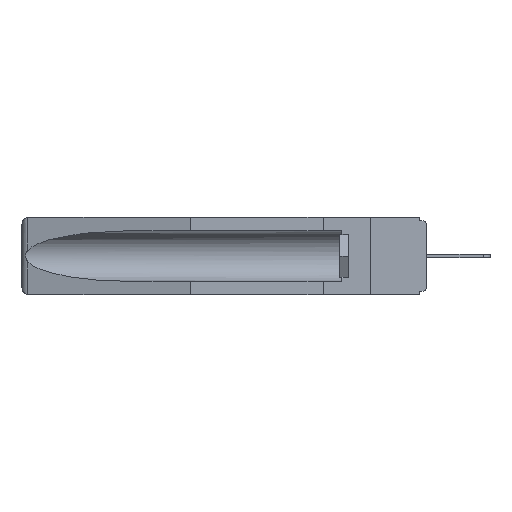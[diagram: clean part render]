
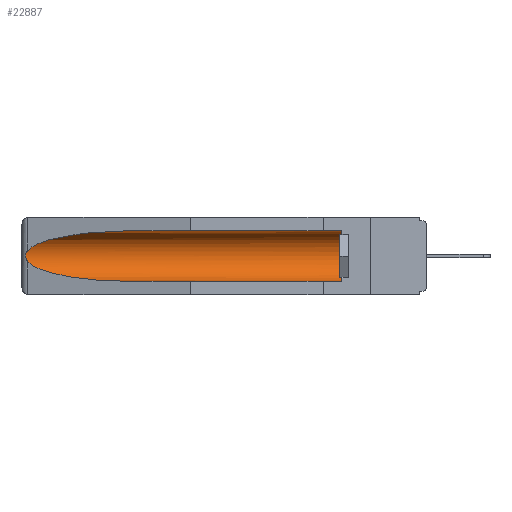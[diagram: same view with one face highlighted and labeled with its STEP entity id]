
A CAD part, left-side view. The second image highlights one B-rep face of the part: STEP entity #22887.
In plain terms, the highlighted cylindrical face has radius 2.857 mm (diameter 5.715 mm), a partial arc.
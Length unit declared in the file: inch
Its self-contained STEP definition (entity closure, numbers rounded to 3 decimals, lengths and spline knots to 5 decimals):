
#917 = CARTESIAN_POINT ( 'NONE',  ( 0.155, -0.30754, -0.1715 ) ) ;
#987 = CARTESIAN_POINT ( 'NONE',  ( 0.2675, 1.53308, -0.16763 ) ) ;
#1352 = CARTESIAN_POINT ( 'NONE',  ( 0.21114, 1.30732, -0.284 ) ) ;
#1881 = ORIENTED_EDGE ( 'NONE', *, *, #13844, .T. ) ;
#3931 = ORIENTED_EDGE ( 'NONE', *, *, #7200, .T. ) ;
#4215 = CARTESIAN_POINT ( 'NONE',  ( 0.26537, 1.52718, -0.19328 ) ) ;
#4476 = DIRECTION ( 'NONE',  ( 0., 1., 0. ) ) ;
#4781 = CARTESIAN_POINT ( 'NONE',  ( 0.155, 0.126, -0.059 ) ) ;
#4835 = EDGE_CURVE ( 'NONE', #23965, #17262, #27785, .T. ) ;
#5038 = VERTEX_POINT ( 'NONE', #23030 ) ;
#5312 = ORIENTED_EDGE ( 'NONE', *, *, #16199, .T. ) ;
#5454 = LINE ( 'NONE', #9443, #24517 ) ;
#5993 = VECTOR ( 'NONE', #4476, 39.37008 ) ;
#6792 = EDGE_LOOP ( 'NONE', ( #22657, #1881, #5312, #8667, #3931, #7073 ) ) ;
#7031 = LINE ( 'NONE', #11035, #5993 ) ;
#7073 = ORIENTED_EDGE ( 'NONE', *, *, #25296, .T. ) ;
#7200 = EDGE_CURVE ( 'NONE', #24203, #20378, #25875, .T. ) ;
#7541 = CARTESIAN_POINT ( 'NONE',  ( 0.26537, 1.52718, -0.19328 ) ) ;
#7619 = DIRECTION ( 'NONE',  ( 0., 0., 1. ) ) ;
#7779 = CARTESIAN_POINT ( 'NONE',  ( 0.25451, 1.48313, -0.24835 ) ) ;
#8667 = ORIENTED_EDGE ( 'NONE', *, *, #20708, .F. ) ;
#9443 = CARTESIAN_POINT ( 'NONE',  ( 0.155, -0.30754, -0.059 ) ) ;
#9468 = CYLINDRICAL_SURFACE ( 'NONE', #20634, 0.1125 ) ;
#9616 = DIRECTION ( 'NONE',  ( 0., 1., 0. ) ) ;
#9686 = CARTESIAN_POINT ( 'NONE',  ( 0.2673, 1.53269, -0.17917 ) ) ;
#10258 = VERTEX_POINT ( 'NONE', #4215 ) ;
#11035 = CARTESIAN_POINT ( 'NONE',  ( 0.155, -0.30754, -0.284 ) ) ;
#11532 = CARTESIAN_POINT ( 'NONE',  ( 0.26597, 1.52961, -0.15275 ) ) ;
#12071 = CARTESIAN_POINT ( 'NONE',  ( 0.21114, 1.30732, -0.059 ) ) ;
#12356 = DIRECTION ( 'NONE',  ( 0., -1., 0. ) ) ;
#13382 = CARTESIAN_POINT ( 'NONE',  ( 0.26654, 1.53092, -0.15636 ) ) ;
#13660 = CARTESIAN_POINT ( 'NONE',  ( 0.155, 0.126, -0.284 ) ) ;
#13801 = CARTESIAN_POINT ( 'NONE',  ( 0.26537, 1.52718, -0.14972 ) ) ;
#13844 = EDGE_CURVE ( 'NONE', #17262, #10258, #16326, .T. ) ;
#13860 = DIRECTION ( 'NONE',  ( 0., 1., 0. ) ) ;
#16199 = EDGE_CURVE ( 'NONE', #10258, #5038, #18138, .T. ) ;
#16209 = CARTESIAN_POINT ( 'NONE',  ( 0.25451, 1.48313, -0.09465 ) ) ;
#16326 = B_SPLINE_CURVE_WITH_KNOTS ( 'NONE', 3,
 ( #18217, #11532, #13382, #27038, #987, #20061, #9686, #17784, #18070, #7541 ),
 .UNSPECIFIED., .F., .F.,
 ( 4, 2, 2, 2, 4 ),
 ( 0., 0.00029, 0.00058, 0.00087, 0.00117 ),
 .UNSPECIFIED. ) ;
#16353 = CARTESIAN_POINT ( 'NONE',  ( 0.155, 1.07973, -0.059 ) ) ;
#17262 = VERTEX_POINT ( 'NONE', #28144 ) ;
#17784 = CARTESIAN_POINT ( 'NONE',  ( 0.26655, 1.53094, -0.18657 ) ) ;
#18070 = CARTESIAN_POINT ( 'NONE',  ( 0.26597, 1.5296, -0.19026 ) ) ;
#18138 =( BOUNDED_CURVE ( )  B_SPLINE_CURVE ( 3, ( #27690, #7779, #1352, #25003 ),
 .UNSPECIFIED., .F., .F. ) 
 B_SPLINE_CURVE_WITH_KNOTS ( ( 4, 4 ),
 ( 0.1948, 1.5708 ),
 .UNSPECIFIED. ) 
 CURVE ( )  GEOMETRIC_REPRESENTATION_ITEM ( )  RATIONAL_B_SPLINE_CURVE ( ( 1., 0.848, 0.848, 1. ) ) 
 REPRESENTATION_ITEM ( '' )  );
#18217 = CARTESIAN_POINT ( 'NONE',  ( 0.26537, 1.52718, -0.14972 ) ) ;
#20061 = CARTESIAN_POINT ( 'NONE',  ( 0.2675, 1.53308, -0.17534 ) ) ;
#20378 = VERTEX_POINT ( 'NONE', #4781 ) ;
#20634 = AXIS2_PLACEMENT_3D ( 'NONE', #917, #9616, #7619 ) ;
#20708 = EDGE_CURVE ( 'NONE', #24203, #5038, #7031, .T. ) ;
#20881 = AXIS2_PLACEMENT_3D ( 'NONE', #25307, #12356, #21038 ) ;
#21038 = DIRECTION ( 'NONE',  ( 0., 0., 1. ) ) ;
#22657 = ORIENTED_EDGE ( 'NONE', *, *, #4835, .T. ) ;
#22850 = FACE_OUTER_BOUND ( 'NONE', #6792, .T. ) ;
#22887 = ADVANCED_FACE ( 'NONE', ( #22850 ), #9468, .F. ) ;
#23030 = CARTESIAN_POINT ( 'NONE',  ( 0.155, 1.07973, -0.284 ) ) ;
#23965 = VERTEX_POINT ( 'NONE', #26582 ) ;
#24203 = VERTEX_POINT ( 'NONE', #13660 ) ;
#24517 = VECTOR ( 'NONE', #13860, 39.37008 ) ;
#25003 = CARTESIAN_POINT ( 'NONE',  ( 0.155, 1.07973, -0.284 ) ) ;
#25296 = EDGE_CURVE ( 'NONE', #20378, #23965, #5454, .T. ) ;
#25307 = CARTESIAN_POINT ( 'NONE',  ( 0.155, 0.126, -0.1715 ) ) ;
#25875 = CIRCLE ( 'NONE', #20881, 0.1125 ) ;
#26582 = CARTESIAN_POINT ( 'NONE',  ( 0.155, 1.07973, -0.059 ) ) ;
#27038 = CARTESIAN_POINT ( 'NONE',  ( 0.2673, 1.5327, -0.16383 ) ) ;
#27690 = CARTESIAN_POINT ( 'NONE',  ( 0.26537, 1.52718, -0.19328 ) ) ;
#27785 =( BOUNDED_CURVE ( )  B_SPLINE_CURVE ( 3, ( #16353, #12071, #16209, #13801 ),
 .UNSPECIFIED., .F., .F. ) 
 B_SPLINE_CURVE_WITH_KNOTS ( ( 4, 4 ),
 ( 4.71239, 6.08839 ),
 .UNSPECIFIED. ) 
 CURVE ( )  GEOMETRIC_REPRESENTATION_ITEM ( )  RATIONAL_B_SPLINE_CURVE ( ( 1., 0.848, 0.848, 1. ) ) 
 REPRESENTATION_ITEM ( '' )  );
#28144 = CARTESIAN_POINT ( 'NONE',  ( 0.26537, 1.52718, -0.14972 ) ) ;
